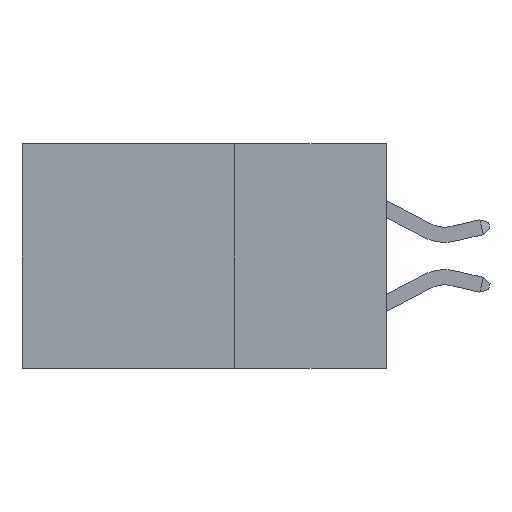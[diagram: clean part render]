
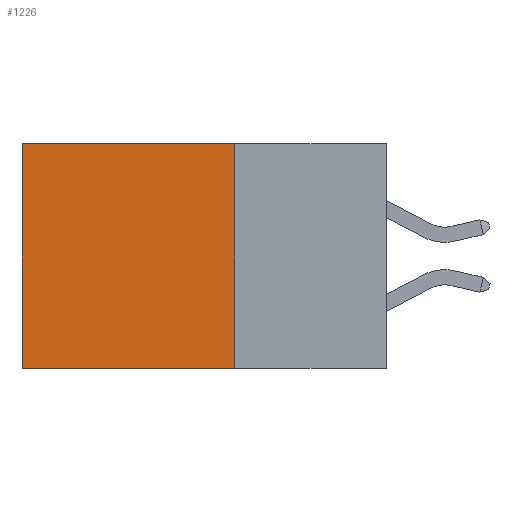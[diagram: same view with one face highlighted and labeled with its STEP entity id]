
A CAD part, left-side view. The second image highlights one B-rep face of the part: STEP entity #1226.
In plain terms, the highlighted planar face has unit normal (-1, 0, 0).
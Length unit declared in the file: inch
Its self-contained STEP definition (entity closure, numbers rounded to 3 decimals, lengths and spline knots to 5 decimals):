
#363 = EDGE_LOOP ( 'NONE', ( #7463, #3260, #9262, #3909 ) ) ;
#372 = DIRECTION ( 'NONE',  ( 0., 0., -1. ) ) ;
#1226 = ADVANCED_FACE ( 'NONE', ( #6168 ), #10941, .F. ) ;
#1835 = CARTESIAN_POINT ( 'NONE',  ( 0.2615, 0.25, -0.37 ) ) ;
#2230 = DIRECTION ( 'NONE',  ( 0., 0., -1. ) ) ;
#2534 = DIRECTION ( 'NONE',  ( 0., 1., 0. ) ) ;
#2566 = VECTOR ( 'NONE', #2534, 39.37008 ) ;
#2616 = CARTESIAN_POINT ( 'NONE',  ( 0.2615, 0.25, -0.37 ) ) ;
#2714 = DIRECTION ( 'NONE',  ( 0., 0., -1. ) ) ;
#2741 = DIRECTION ( 'NONE',  ( 1., 0., 0. ) ) ;
#3260 = ORIENTED_EDGE ( 'NONE', *, *, #3509, .F. ) ;
#3296 = CARTESIAN_POINT ( 'NONE',  ( 0.2615, 0.25, -0.37 ) ) ;
#3509 = EDGE_CURVE ( 'NONE', #11619, #3602, #5394, .T. ) ;
#3602 = VERTEX_POINT ( 'NONE', #7701 ) ;
#3909 = ORIENTED_EDGE ( 'NONE', *, *, #8990, .T. ) ;
#4820 = DIRECTION ( 'NONE',  ( 0., 1., 0. ) ) ;
#4898 = CARTESIAN_POINT ( 'NONE',  ( 0.2615, 0.25, 0. ) ) ;
#5394 = LINE ( 'NONE', #2616, #2566 ) ;
#5422 = VECTOR ( 'NONE', #372, 39.37008 ) ;
#5570 = CARTESIAN_POINT ( 'NONE',  ( 0.2615, 0.6, 0. ) ) ;
#6168 = FACE_OUTER_BOUND ( 'NONE', #363, .T. ) ;
#6469 = CARTESIAN_POINT ( 'NONE',  ( 0.2615, 0.6, -0.37 ) ) ;
#7348 = VERTEX_POINT ( 'NONE', #12659 ) ;
#7463 = ORIENTED_EDGE ( 'NONE', *, *, #9616, .T. ) ;
#7701 = CARTESIAN_POINT ( 'NONE',  ( 0.2615, 0.6, -0.37 ) ) ;
#7716 = CARTESIAN_POINT ( 'NONE',  ( 0.2615, 0.25, -0.37 ) ) ;
#7742 = VERTEX_POINT ( 'NONE', #5570 ) ;
#7976 = VECTOR ( 'NONE', #4820, 39.37008 ) ;
#8990 = EDGE_CURVE ( 'NONE', #7348, #7742, #12849, .T. ) ;
#9262 = ORIENTED_EDGE ( 'NONE', *, *, #10604, .F. ) ;
#9616 = EDGE_CURVE ( 'NONE', #7742, #3602, #11623, .T. ) ;
#10604 = EDGE_CURVE ( 'NONE', #7348, #11619, #12437, .T. ) ;
#10941 = PLANE ( 'NONE',  #12453 ) ;
#11061 = VECTOR ( 'NONE', #2230, 39.37008 ) ;
#11619 = VERTEX_POINT ( 'NONE', #1835 ) ;
#11623 = LINE ( 'NONE', #6469, #11061 ) ;
#12437 = LINE ( 'NONE', #7716, #5422 ) ;
#12453 = AXIS2_PLACEMENT_3D ( 'NONE', #3296, #2741, #2714 ) ;
#12659 = CARTESIAN_POINT ( 'NONE',  ( 0.2615, 0.25, 0. ) ) ;
#12849 = LINE ( 'NONE', #4898, #7976 ) ;
